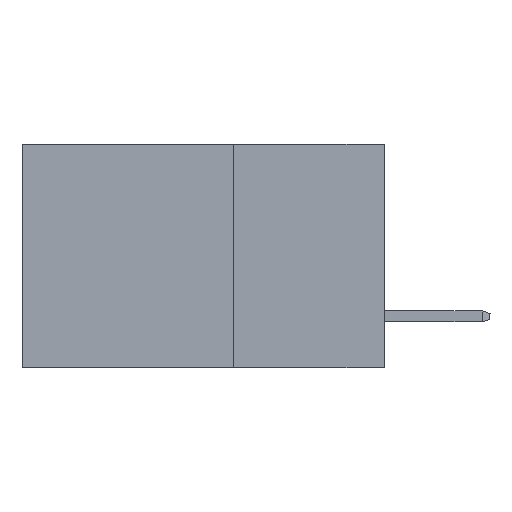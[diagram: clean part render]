
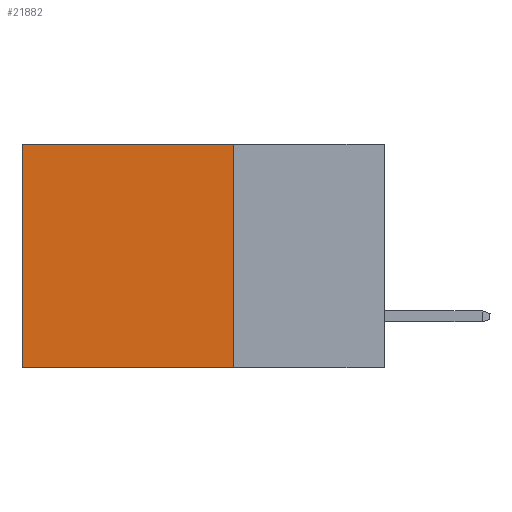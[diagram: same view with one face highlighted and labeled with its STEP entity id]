
A CAD part, left-side view. The second image highlights one B-rep face of the part: STEP entity #21882.
In plain terms, the highlighted planar face has unit normal (-1, 0, 0).
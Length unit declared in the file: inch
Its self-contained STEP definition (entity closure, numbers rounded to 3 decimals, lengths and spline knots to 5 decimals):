
#8 = ORIENTED_EDGE ( 'NONE', *, *, #5241, .T. ) ;
#700 = ORIENTED_EDGE ( 'NONE', *, *, #19611, .F. ) ;
#1217 = CARTESIAN_POINT ( 'NONE',  ( 0.2615, 0.6, -0.37 ) ) ;
#1331 = ORIENTED_EDGE ( 'NONE', *, *, #6277, .F. ) ;
#4399 = VECTOR ( 'NONE', #24872, 39.37008 ) ;
#4592 = VERTEX_POINT ( 'NONE', #7667 ) ;
#4973 = AXIS2_PLACEMENT_3D ( 'NONE', #17620, #5986, #19552 ) ;
#5241 = EDGE_CURVE ( 'NONE', #9837, #4592, #24898, .T. ) ;
#5788 = VECTOR ( 'NONE', #8107, 39.37008 ) ;
#5986 = DIRECTION ( 'NONE',  ( 1., 0., 0. ) ) ;
#6102 = CARTESIAN_POINT ( 'NONE',  ( 0.2615, 0.6, 0. ) ) ;
#6277 = EDGE_CURVE ( 'NONE', #12870, #13177, #8585, .T. ) ;
#7667 = CARTESIAN_POINT ( 'NONE',  ( 0.2615, 0.6, -0.37 ) ) ;
#7827 = LINE ( 'NONE', #9072, #22681 ) ;
#8107 = DIRECTION ( 'NONE',  ( 0., 1., 0. ) ) ;
#8232 = CARTESIAN_POINT ( 'NONE',  ( 0.2615, 0.25, 0. ) ) ;
#8585 = LINE ( 'NONE', #19168, #13753 ) ;
#9072 = CARTESIAN_POINT ( 'NONE',  ( 0.2615, 0.25, -0.37 ) ) ;
#9837 = VERTEX_POINT ( 'NONE', #6102 ) ;
#9891 = CARTESIAN_POINT ( 'NONE',  ( 0.2615, 0.25, -0.37 ) ) ;
#11633 = FACE_OUTER_BOUND ( 'NONE', #19610, .T. ) ;
#12870 = VERTEX_POINT ( 'NONE', #19996 ) ;
#13177 = VERTEX_POINT ( 'NONE', #9891 ) ;
#13753 = VECTOR ( 'NONE', #19094, 39.37008 ) ;
#15042 = EDGE_CURVE ( 'NONE', #12870, #9837, #16139, .T. ) ;
#15686 = PLANE ( 'NONE',  #4973 ) ;
#16139 = LINE ( 'NONE', #8232, #5788 ) ;
#17620 = CARTESIAN_POINT ( 'NONE',  ( 0.2615, 0.25, -0.37 ) ) ;
#18712 = DIRECTION ( 'NONE',  ( 0., 1., 0. ) ) ;
#19094 = DIRECTION ( 'NONE',  ( 0., 0., -1. ) ) ;
#19168 = CARTESIAN_POINT ( 'NONE',  ( 0.2615, 0.25, -0.37 ) ) ;
#19552 = DIRECTION ( 'NONE',  ( 0., 0., -1. ) ) ;
#19610 = EDGE_LOOP ( 'NONE', ( #8, #700, #1331, #19892 ) ) ;
#19611 = EDGE_CURVE ( 'NONE', #13177, #4592, #7827, .T. ) ;
#19892 = ORIENTED_EDGE ( 'NONE', *, *, #15042, .T. ) ;
#19996 = CARTESIAN_POINT ( 'NONE',  ( 0.2615, 0.25, 0. ) ) ;
#21882 = ADVANCED_FACE ( 'NONE', ( #11633 ), #15686, .F. ) ;
#22681 = VECTOR ( 'NONE', #18712, 39.37008 ) ;
#24872 = DIRECTION ( 'NONE',  ( 0., 0., -1. ) ) ;
#24898 = LINE ( 'NONE', #1217, #4399 ) ;
